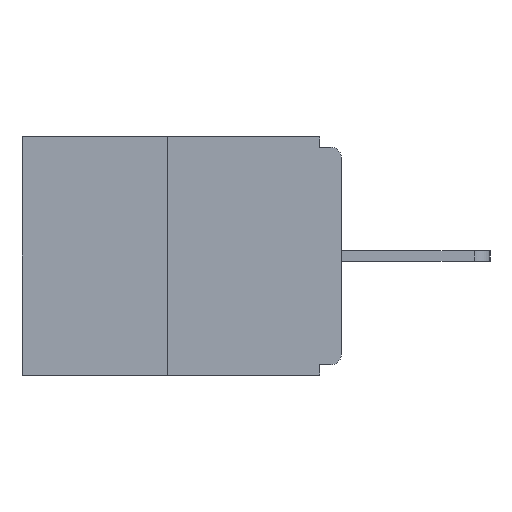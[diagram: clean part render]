
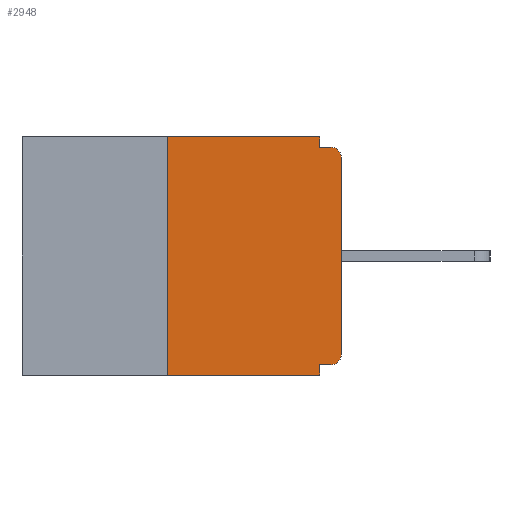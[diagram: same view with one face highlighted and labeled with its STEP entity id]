
A CAD part, left-side view. The second image highlights one B-rep face of the part: STEP entity #2948.
In plain terms, the highlighted planar face has unit normal (-1, 0, 0).
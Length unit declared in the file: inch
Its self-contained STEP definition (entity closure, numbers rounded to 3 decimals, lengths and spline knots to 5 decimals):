
#561 = EDGE_CURVE ( 'NONE', #10698, #8714, #10816, .T. ) ;
#627 = DIRECTION ( 'NONE',  ( -1., 0., 0. ) ) ;
#1742 = CARTESIAN_POINT ( 'NONE',  ( 0., 0., -0.03 ) ) ;
#2021 = DIRECTION ( 'NONE',  ( 0., 0., 1. ) ) ;
#2056 = CARTESIAN_POINT ( 'NONE',  ( 0., 0., 0. ) ) ;
#2084 = AXIS2_PLACEMENT_3D ( 'NONE', #7126, #7168, #7157 ) ;
#2316 = VERTEX_POINT ( 'NONE', #10308 ) ;
#2375 = VERTEX_POINT ( 'NONE', #6096 ) ;
#2394 = LINE ( 'NONE', #5057, #13175 ) ;
#2441 = VERTEX_POINT ( 'NONE', #3939 ) ;
#2492 = LINE ( 'NONE', #4241, #13255 ) ;
#2788 = VECTOR ( 'NONE', #9859, 39.37008 ) ;
#2856 = VERTEX_POINT ( 'NONE', #11930 ) ;
#2871 = CIRCLE ( 'NONE', #13113, 0.015 ) ;
#2921 = VERTEX_POINT ( 'NONE', #11529 ) ;
#2948 = ADVANCED_FACE ( 'NONE', ( #3834 ), #7720, .F. ) ;
#2998 = CARTESIAN_POINT ( 'NONE',  ( 0., 0.015, -0.03 ) ) ;
#3524 = CARTESIAN_POINT ( 'NONE',  ( 0., 0.015, -0.015 ) ) ;
#3834 = FACE_OUTER_BOUND ( 'NONE', #10864, .T. ) ;
#3867 = ORIENTED_EDGE ( 'NONE', *, *, #561, .T. ) ;
#3939 = CARTESIAN_POINT ( 'NONE',  ( 0., 0.031, -0.015 ) ) ;
#4241 = CARTESIAN_POINT ( 'NONE',  ( 0., 0.031, 0. ) ) ;
#4371 = ORIENTED_EDGE ( 'NONE', *, *, #12531, .F. ) ;
#4548 = DIRECTION ( 'NONE',  ( 0., -1., 0. ) ) ;
#5057 = CARTESIAN_POINT ( 'NONE',  ( 0., 0.46, -0.343 ) ) ;
#5177 = EDGE_CURVE ( 'NONE', #2375, #2921, #7383, .T. ) ;
#5367 = EDGE_CURVE ( 'NONE', #9712, #2856, #13615, .T. ) ;
#5649 = EDGE_CURVE ( 'NONE', #9712, #2921, #2394, .T. ) ;
#5897 = LINE ( 'NONE', #12718, #2788 ) ;
#6003 = CARTESIAN_POINT ( 'NONE',  ( 0., 0.015, -0.328 ) ) ;
#6055 = VECTOR ( 'NONE', #8115, 39.37008 ) ;
#6080 = DIRECTION ( 'NONE',  ( 0., 1., 0. ) ) ;
#6096 = CARTESIAN_POINT ( 'NONE',  ( 0., 0.031, -0.328 ) ) ;
#6107 = CARTESIAN_POINT ( 'NONE',  ( 0., 0., -0.328 ) ) ;
#7126 = CARTESIAN_POINT ( 'NONE',  ( 0., 0.46, 0. ) ) ;
#7157 = DIRECTION ( 'NONE',  ( 0., 0., -1. ) ) ;
#7168 = DIRECTION ( 'NONE',  ( 1., 0., 0. ) ) ;
#7383 = LINE ( 'NONE', #9297, #12286 ) ;
#7493 = ORIENTED_EDGE ( 'NONE', *, *, #5649, .T. ) ;
#7563 = DIRECTION ( 'NONE',  ( 0., 0., -1. ) ) ;
#7604 = CARTESIAN_POINT ( 'NONE',  ( 0., 0.015, -0.313 ) ) ;
#7720 = PLANE ( 'NONE',  #2084 ) ;
#7833 = EDGE_CURVE ( 'NONE', #2441, #8714, #8278, .T. ) ;
#7909 = VECTOR ( 'NONE', #2021, 39.37008 ) ;
#7923 = CARTESIAN_POINT ( 'NONE',  ( 0., 0.25, 0. ) ) ;
#7939 = VECTOR ( 'NONE', #9107, 39.37008 ) ;
#8115 = DIRECTION ( 'NONE',  ( 0., 0., 1. ) ) ;
#8278 = LINE ( 'NONE', #9119, #7939 ) ;
#8368 = EDGE_CURVE ( 'NONE', #8398, #2375, #11468, .T. ) ;
#8398 = VERTEX_POINT ( 'NONE', #6003 ) ;
#8589 = VECTOR ( 'NONE', #6080, 39.37008 ) ;
#8637 = DIRECTION ( 'NONE',  ( 0., 0., -1. ) ) ;
#8714 = VERTEX_POINT ( 'NONE', #3524 ) ;
#8955 = EDGE_CURVE ( 'NONE', #2316, #10698, #13104, .T. ) ;
#9107 = DIRECTION ( 'NONE',  ( 0., -1., 0. ) ) ;
#9119 = CARTESIAN_POINT ( 'NONE',  ( 0., 0., -0.015 ) ) ;
#9271 = DIRECTION ( 'NONE',  ( 0., 0., -1. ) ) ;
#9297 = CARTESIAN_POINT ( 'NONE',  ( 0., 0.031, -0.343 ) ) ;
#9334 = ORIENTED_EDGE ( 'NONE', *, *, #8955, .T. ) ;
#9712 = VERTEX_POINT ( 'NONE', #10249 ) ;
#9859 = DIRECTION ( 'NONE',  ( 0., -1., 0. ) ) ;
#10187 = ORIENTED_EDGE ( 'NONE', *, *, #7833, .F. ) ;
#10249 = CARTESIAN_POINT ( 'NONE',  ( 0., 0.25, -0.343 ) ) ;
#10308 = CARTESIAN_POINT ( 'NONE',  ( 0., 0., -0.313 ) ) ;
#10373 = AXIS2_PLACEMENT_3D ( 'NONE', #2998, #11503, #13344 ) ;
#10698 = VERTEX_POINT ( 'NONE', #1742 ) ;
#10816 = CIRCLE ( 'NONE', #10373, 0.015 ) ;
#10864 = EDGE_LOOP ( 'NONE', ( #4371, #10875, #7493, #11360, #11086, #12429, #9334, #3867, #10187, #11185 ) ) ;
#10875 = ORIENTED_EDGE ( 'NONE', *, *, #5367, .F. ) ;
#11086 = ORIENTED_EDGE ( 'NONE', *, *, #8368, .F. ) ;
#11185 = ORIENTED_EDGE ( 'NONE', *, *, #13049, .F. ) ;
#11314 = VERTEX_POINT ( 'NONE', #13072 ) ;
#11360 = ORIENTED_EDGE ( 'NONE', *, *, #5177, .F. ) ;
#11468 = LINE ( 'NONE', #6107, #8589 ) ;
#11503 = DIRECTION ( 'NONE',  ( -1., 0., 0. ) ) ;
#11529 = CARTESIAN_POINT ( 'NONE',  ( 0., 0.031, -0.343 ) ) ;
#11930 = CARTESIAN_POINT ( 'NONE',  ( 0., 0.25, 0. ) ) ;
#12286 = VECTOR ( 'NONE', #9271, 39.37008 ) ;
#12429 = ORIENTED_EDGE ( 'NONE', *, *, #13071, .T. ) ;
#12531 = EDGE_CURVE ( 'NONE', #2856, #11314, #5897, .T. ) ;
#12718 = CARTESIAN_POINT ( 'NONE',  ( 0., 0.46, 0. ) ) ;
#13049 = EDGE_CURVE ( 'NONE', #11314, #2441, #2492, .T. ) ;
#13071 = EDGE_CURVE ( 'NONE', #8398, #2316, #2871, .T. ) ;
#13072 = CARTESIAN_POINT ( 'NONE',  ( 0., 0.031, 0. ) ) ;
#13104 = LINE ( 'NONE', #2056, #7909 ) ;
#13113 = AXIS2_PLACEMENT_3D ( 'NONE', #7604, #627, #8637 ) ;
#13175 = VECTOR ( 'NONE', #4548, 39.37008 ) ;
#13255 = VECTOR ( 'NONE', #7563, 39.37008 ) ;
#13344 = DIRECTION ( 'NONE',  ( 0., 0., -1. ) ) ;
#13615 = LINE ( 'NONE', #7923, #6055 ) ;
